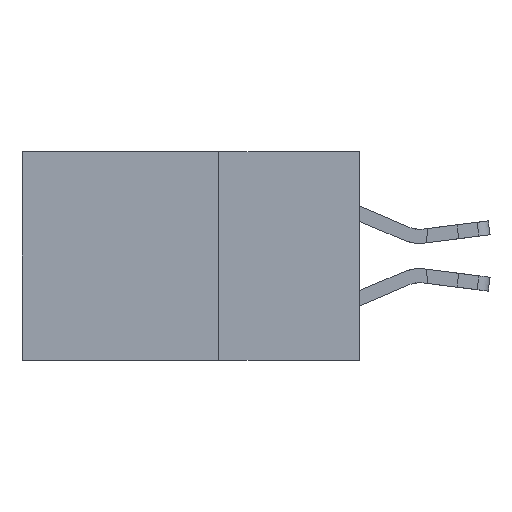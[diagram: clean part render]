
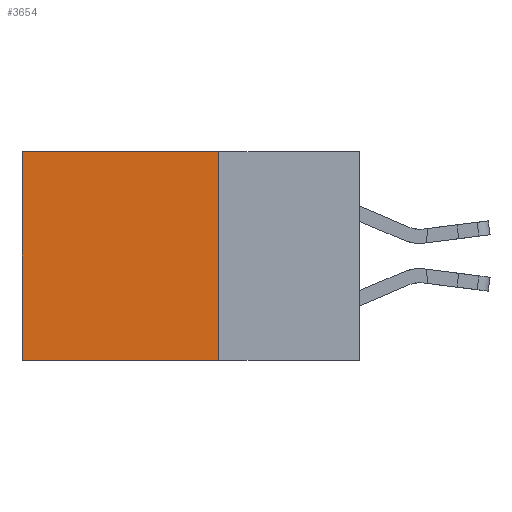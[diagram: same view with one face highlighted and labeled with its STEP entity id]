
A CAD part, left-side view. The second image highlights one B-rep face of the part: STEP entity #3654.
In plain terms, the highlighted planar face has unit normal (-1, 0, 0).
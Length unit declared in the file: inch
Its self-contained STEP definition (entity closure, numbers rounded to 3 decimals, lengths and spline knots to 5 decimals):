
#814 = DIRECTION ( 'NONE',  ( 0., 0., -1. ) ) ;
#973 = CARTESIAN_POINT ( 'NONE',  ( 0.2875, 0.25, -0.37 ) ) ;
#1029 = VERTEX_POINT ( 'NONE', #5770 ) ;
#1471 = CARTESIAN_POINT ( 'NONE',  ( 0.2875, 0.25, 0. ) ) ;
#2377 = EDGE_CURVE ( 'NONE', #2814, #3940, #9304, .T. ) ;
#2814 = VERTEX_POINT ( 'NONE', #3500 ) ;
#3195 = ORIENTED_EDGE ( 'NONE', *, *, #5845, .T. ) ;
#3500 = CARTESIAN_POINT ( 'NONE',  ( 0.2875, 0.25, 0. ) ) ;
#3579 = LINE ( 'NONE', #973, #8848 ) ;
#3654 = ADVANCED_FACE ( 'NONE', ( #5265 ), #13031, .F. ) ;
#3814 = CARTESIAN_POINT ( 'NONE',  ( 0.2875, 0.25, 0. ) ) ;
#3940 = VERTEX_POINT ( 'NONE', #6114 ) ;
#4204 = DIRECTION ( 'NONE',  ( 1., 0., 0. ) ) ;
#5265 = FACE_OUTER_BOUND ( 'NONE', #10419, .T. ) ;
#5386 = DIRECTION ( 'NONE',  ( 0., 1., 0. ) ) ;
#5770 = CARTESIAN_POINT ( 'NONE',  ( 0.2875, 0.25, -0.37 ) ) ;
#5845 = EDGE_CURVE ( 'NONE', #3940, #17749, #18602, .T. ) ;
#6025 = LINE ( 'NONE', #3814, #10843 ) ;
#6114 = CARTESIAN_POINT ( 'NONE',  ( 0.2875, 0.6, 0. ) ) ;
#6397 = EDGE_CURVE ( 'NONE', #2814, #1029, #6025, .T. ) ;
#6824 = ORIENTED_EDGE ( 'NONE', *, *, #2377, .T. ) ;
#7072 = CARTESIAN_POINT ( 'NONE',  ( 0.2875, 0.25, 0. ) ) ;
#8733 = DIRECTION ( 'NONE',  ( 0., 0., -1. ) ) ;
#8848 = VECTOR ( 'NONE', #5386, 39.37008 ) ;
#9304 = LINE ( 'NONE', #1471, #15446 ) ;
#9482 = EDGE_CURVE ( 'NONE', #1029, #17749, #3579, .T. ) ;
#10035 = AXIS2_PLACEMENT_3D ( 'NONE', #7072, #4204, #8733 ) ;
#10419 = EDGE_LOOP ( 'NONE', ( #3195, #15442, #17731, #6824 ) ) ;
#10843 = VECTOR ( 'NONE', #814, 39.37008 ) ;
#11190 = CARTESIAN_POINT ( 'NONE',  ( 0.2875, 0.6, -0.37 ) ) ;
#11329 = DIRECTION ( 'NONE',  ( 0., 0., -1. ) ) ;
#13031 = PLANE ( 'NONE',  #10035 ) ;
#14585 = DIRECTION ( 'NONE',  ( 0., 1., 0. ) ) ;
#15414 = VECTOR ( 'NONE', #11329, 39.37008 ) ;
#15442 = ORIENTED_EDGE ( 'NONE', *, *, #9482, .F. ) ;
#15446 = VECTOR ( 'NONE', #14585, 39.37008 ) ;
#17731 = ORIENTED_EDGE ( 'NONE', *, *, #6397, .F. ) ;
#17749 = VERTEX_POINT ( 'NONE', #11190 ) ;
#18311 = CARTESIAN_POINT ( 'NONE',  ( 0.2875, 0.6, 0. ) ) ;
#18602 = LINE ( 'NONE', #18311, #15414 ) ;
